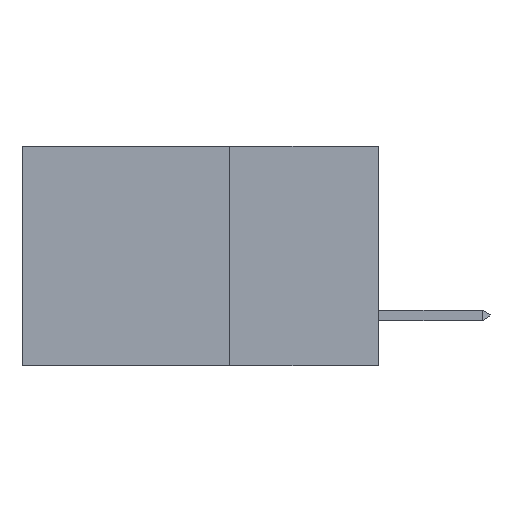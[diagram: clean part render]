
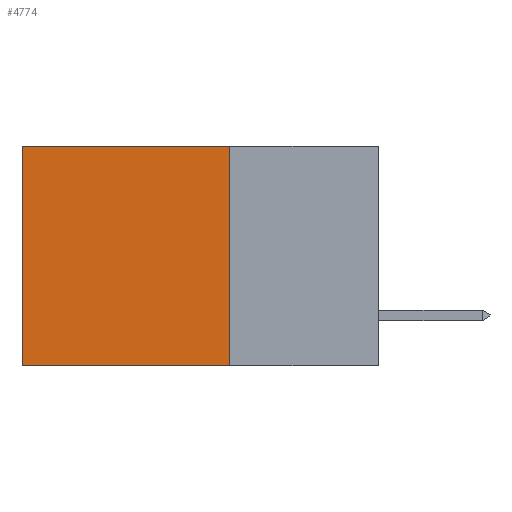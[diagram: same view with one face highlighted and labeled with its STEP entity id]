
A CAD part, left-side view. The second image highlights one B-rep face of the part: STEP entity #4774.
In plain terms, the highlighted planar face has unit normal (-1, 0, 0).
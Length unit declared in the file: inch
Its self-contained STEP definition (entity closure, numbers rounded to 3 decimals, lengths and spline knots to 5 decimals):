
#348 = CARTESIAN_POINT ( 'NONE',  ( 0.2615, 0.25, 0. ) ) ;
#403 = EDGE_LOOP ( 'NONE', ( #7771, #4068, #5472, #8748 ) ) ;
#466 = DIRECTION ( 'NONE',  ( 0., 1., 0. ) ) ;
#616 = DIRECTION ( 'NONE',  ( 0., 0., -1. ) ) ;
#753 = VERTEX_POINT ( 'NONE', #2654 ) ;
#794 = AXIS2_PLACEMENT_3D ( 'NONE', #6744, #7505, #4436 ) ;
#1101 = VERTEX_POINT ( 'NONE', #3218 ) ;
#1319 = DIRECTION ( 'NONE',  ( 0., 0., -1. ) ) ;
#1432 = VECTOR ( 'NONE', #466, 39.37008 ) ;
#2035 = CARTESIAN_POINT ( 'NONE',  ( 0.2615, 0.6, -0.37 ) ) ;
#2114 = LINE ( 'NONE', #5246, #1432 ) ;
#2401 = LINE ( 'NONE', #4096, #7414 ) ;
#2562 = EDGE_CURVE ( 'NONE', #753, #1101, #5232, .T. ) ;
#2654 = CARTESIAN_POINT ( 'NONE',  ( 0.2615, 0.25, 0. ) ) ;
#2950 = VERTEX_POINT ( 'NONE', #2035 ) ;
#3218 = CARTESIAN_POINT ( 'NONE',  ( 0.2615, 0.25, -0.37 ) ) ;
#3486 = DIRECTION ( 'NONE',  ( 0., 1., 0. ) ) ;
#3512 = VERTEX_POINT ( 'NONE', #5599 ) ;
#4068 = ORIENTED_EDGE ( 'NONE', *, *, #9689, .F. ) ;
#4096 = CARTESIAN_POINT ( 'NONE',  ( 0.2615, 0.6, -0.37 ) ) ;
#4436 = DIRECTION ( 'NONE',  ( 0., 0., -1. ) ) ;
#4611 = CARTESIAN_POINT ( 'NONE',  ( 0.2615, 0.25, -0.37 ) ) ;
#4774 = ADVANCED_FACE ( 'NONE', ( #8792 ), #7253, .F. ) ;
#4873 = VECTOR ( 'NONE', #3486, 39.37008 ) ;
#5090 = VECTOR ( 'NONE', #1319, 39.37008 ) ;
#5232 = LINE ( 'NONE', #4611, #5090 ) ;
#5246 = CARTESIAN_POINT ( 'NONE',  ( 0.2615, 0.25, -0.37 ) ) ;
#5472 = ORIENTED_EDGE ( 'NONE', *, *, #2562, .F. ) ;
#5599 = CARTESIAN_POINT ( 'NONE',  ( 0.2615, 0.6, 0. ) ) ;
#6744 = CARTESIAN_POINT ( 'NONE',  ( 0.2615, 0.25, -0.37 ) ) ;
#7253 = PLANE ( 'NONE',  #794 ) ;
#7369 = LINE ( 'NONE', #348, #4873 ) ;
#7414 = VECTOR ( 'NONE', #616, 39.37008 ) ;
#7505 = DIRECTION ( 'NONE',  ( 1., 0., 0. ) ) ;
#7771 = ORIENTED_EDGE ( 'NONE', *, *, #8496, .T. ) ;
#8496 = EDGE_CURVE ( 'NONE', #3512, #2950, #2401, .T. ) ;
#8748 = ORIENTED_EDGE ( 'NONE', *, *, #9991, .T. ) ;
#8792 = FACE_OUTER_BOUND ( 'NONE', #403, .T. ) ;
#9689 = EDGE_CURVE ( 'NONE', #1101, #2950, #2114, .T. ) ;
#9991 = EDGE_CURVE ( 'NONE', #753, #3512, #7369, .T. ) ;
